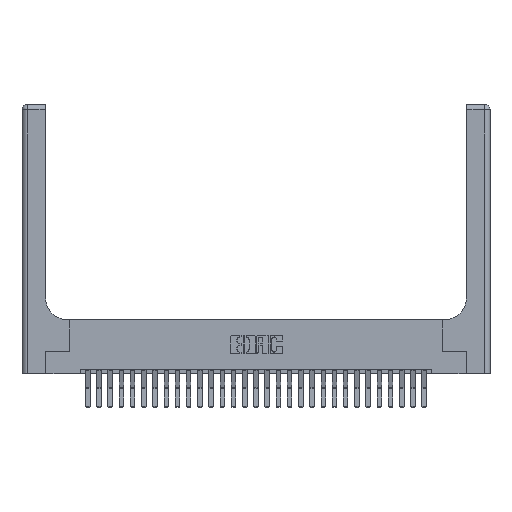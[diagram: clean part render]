
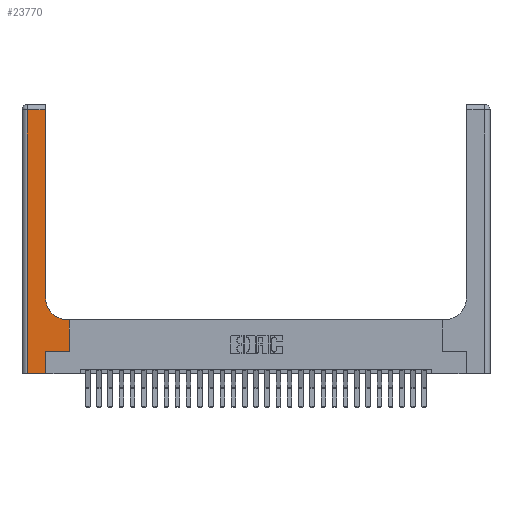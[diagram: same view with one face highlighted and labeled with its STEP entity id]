
A CAD part, top view. The second image highlights one B-rep face of the part: STEP entity #23770.
In plain terms, the highlighted planar face has unit normal (0, 0, 1).
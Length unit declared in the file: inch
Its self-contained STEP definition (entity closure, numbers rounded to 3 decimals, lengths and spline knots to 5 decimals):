
#694 = CARTESIAN_POINT ( 'NONE',  ( 0.26, 0.85, 0.37 ) ) ;
#938 = CARTESIAN_POINT ( 'NONE',  ( 0.06, 3., 0.37 ) ) ;
#1077 = PLANE ( 'NONE',  #20285 ) ;
#2193 = CARTESIAN_POINT ( 'NONE',  ( 0.265, 0., 0.37 ) ) ;
#2479 = CARTESIAN_POINT ( 'NONE',  ( 0.528, 0.25, 0.37 ) ) ;
#2490 = DIRECTION ( 'NONE',  ( 0., -1., 0. ) ) ;
#2688 = VECTOR ( 'NONE', #19669, 39.37008 ) ;
#3255 = EDGE_CURVE ( 'NONE', #20485, #8542, #21487, .T. ) ;
#3284 = LINE ( 'NONE', #9151, #2688 ) ;
#3516 = VECTOR ( 'NONE', #2490, 39.37008 ) ;
#4246 = CARTESIAN_POINT ( 'NONE',  ( 0.528, 0.6, 0.37 ) ) ;
#4486 = EDGE_CURVE ( 'NONE', #22393, #20485, #26691, .T. ) ;
#5464 = CARTESIAN_POINT ( 'NONE',  ( 0.51, 0.85, 0.37 ) ) ;
#5571 = VECTOR ( 'NONE', #20432, 39.37008 ) ;
#6636 = LINE ( 'NONE', #11091, #22159 ) ;
#6772 = EDGE_CURVE ( 'NONE', #9771, #18141, #6636, .T. ) ;
#6898 = ORIENTED_EDGE ( 'NONE', *, *, #15040, .T. ) ;
#6942 = EDGE_CURVE ( 'NONE', #18141, #22393, #3284, .T. ) ;
#7515 = ORIENTED_EDGE ( 'NONE', *, *, #21464, .T. ) ;
#7816 = LINE ( 'NONE', #22226, #5571 ) ;
#7827 = VECTOR ( 'NONE', #11102, 39.37008 ) ;
#8142 = CARTESIAN_POINT ( 'NONE',  ( 0.26, 0.6, 0.37 ) ) ;
#8326 = DIRECTION ( 'NONE',  ( 1., 0., 0. ) ) ;
#8542 = VERTEX_POINT ( 'NONE', #4246 ) ;
#8896 = LINE ( 'NONE', #938, #3516 ) ;
#9151 = CARTESIAN_POINT ( 'NONE',  ( 0.265, 0., 0.37 ) ) ;
#9748 = CARTESIAN_POINT ( 'NONE',  ( 0.06, 0., 0.37 ) ) ;
#9771 = VERTEX_POINT ( 'NONE', #9748 ) ;
#9956 = CARTESIAN_POINT ( 'NONE',  ( 0., 2.94, 0.37 ) ) ;
#11091 = CARTESIAN_POINT ( 'NONE',  ( 0., 0., 0.37 ) ) ;
#11102 = DIRECTION ( 'NONE',  ( 0., 1., 0. ) ) ;
#11797 = DIRECTION ( 'NONE',  ( -1., 0., 0. ) ) ;
#12827 = EDGE_CURVE ( 'NONE', #8542, #22100, #24516, .T. ) ;
#12914 = CARTESIAN_POINT ( 'NONE',  ( 0.51, 0.6, 0.37 ) ) ;
#14141 = EDGE_LOOP ( 'NONE', ( #6898, #22711, #24143, #18552, #17695, #14813, #15206, #16901, #7515 ) ) ;
#14471 = CIRCLE ( 'NONE', #24649, 0.25 ) ;
#14813 = ORIENTED_EDGE ( 'NONE', *, *, #4486, .T. ) ;
#15040 = EDGE_CURVE ( 'NONE', #19145, #21273, #7816, .T. ) ;
#15206 = ORIENTED_EDGE ( 'NONE', *, *, #3255, .T. ) ;
#15904 = DIRECTION ( 'NONE',  ( 0., 0., -1. ) ) ;
#15978 = CARTESIAN_POINT ( 'NONE',  ( 0., 3., 0.37 ) ) ;
#16238 = VERTEX_POINT ( 'NONE', #26011 ) ;
#16491 = DIRECTION ( 'NONE',  ( -1., 0., 0. ) ) ;
#16747 = DIRECTION ( 'NONE',  ( -1., 0., 0. ) ) ;
#16901 = ORIENTED_EDGE ( 'NONE', *, *, #12827, .T. ) ;
#17015 = CARTESIAN_POINT ( 'NONE',  ( 0.265, 0.25, 0.37 ) ) ;
#17695 = ORIENTED_EDGE ( 'NONE', *, *, #6942, .T. ) ;
#17698 = VECTOR ( 'NONE', #16747, 39.37008 ) ;
#18141 = VERTEX_POINT ( 'NONE', #2193 ) ;
#18174 = DIRECTION ( 'NONE',  ( 0., 0., -1. ) ) ;
#18552 = ORIENTED_EDGE ( 'NONE', *, *, #6772, .T. ) ;
#18726 = CARTESIAN_POINT ( 'NONE',  ( 0.528, 0.25, 0.37 ) ) ;
#18811 = LINE ( 'NONE', #9956, #17698 ) ;
#19145 = VERTEX_POINT ( 'NONE', #694 ) ;
#19533 = DIRECTION ( 'NONE',  ( 1., 0., 0. ) ) ;
#19669 = DIRECTION ( 'NONE',  ( 0., 1., 0. ) ) ;
#20097 = FACE_OUTER_BOUND ( 'NONE', #14141, .T. ) ;
#20285 = AXIS2_PLACEMENT_3D ( 'NONE', #15978, #18174, #11797 ) ;
#20432 = DIRECTION ( 'NONE',  ( 0., 1., 0. ) ) ;
#20485 = VERTEX_POINT ( 'NONE', #18726 ) ;
#21273 = VERTEX_POINT ( 'NONE', #21429 ) ;
#21429 = CARTESIAN_POINT ( 'NONE',  ( 0.26, 2.94, 0.37 ) ) ;
#21434 = VECTOR ( 'NONE', #16491, 39.37008 ) ;
#21464 = EDGE_CURVE ( 'NONE', #22100, #19145, #14471, .T. ) ;
#21487 = LINE ( 'NONE', #2479, #7827 ) ;
#22100 = VERTEX_POINT ( 'NONE', #12914 ) ;
#22159 = VECTOR ( 'NONE', #19533, 39.37008 ) ;
#22226 = CARTESIAN_POINT ( 'NONE',  ( 0.26, 3., 0.37 ) ) ;
#22393 = VERTEX_POINT ( 'NONE', #17015 ) ;
#22711 = ORIENTED_EDGE ( 'NONE', *, *, #24377, .T. ) ;
#22800 = VECTOR ( 'NONE', #8326, 39.37008 ) ;
#23770 = ADVANCED_FACE ( 'NONE', ( #20097 ), #1077, .F. ) ;
#24143 = ORIENTED_EDGE ( 'NONE', *, *, #25278, .T. ) ;
#24333 = DIRECTION ( 'NONE',  ( 1., 0., 0. ) ) ;
#24377 = EDGE_CURVE ( 'NONE', #21273, #16238, #18811, .T. ) ;
#24516 = LINE ( 'NONE', #8142, #21434 ) ;
#24649 = AXIS2_PLACEMENT_3D ( 'NONE', #5464, #15904, #24333 ) ;
#25242 = CARTESIAN_POINT ( 'NONE',  ( 0.265, 0.25, 0.37 ) ) ;
#25278 = EDGE_CURVE ( 'NONE', #16238, #9771, #8896, .T. ) ;
#26011 = CARTESIAN_POINT ( 'NONE',  ( 0.06, 2.94, 0.37 ) ) ;
#26691 = LINE ( 'NONE', #25242, #22800 ) ;
